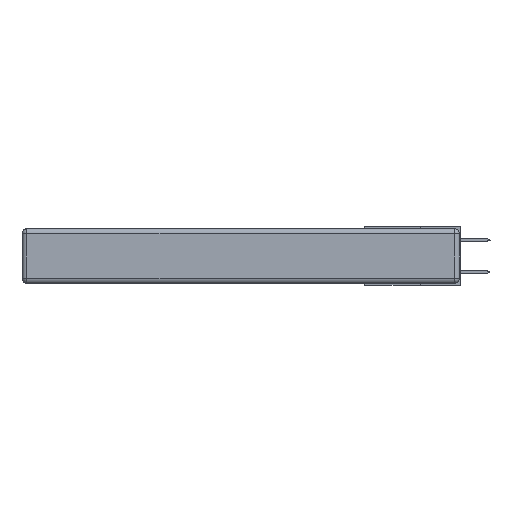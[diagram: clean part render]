
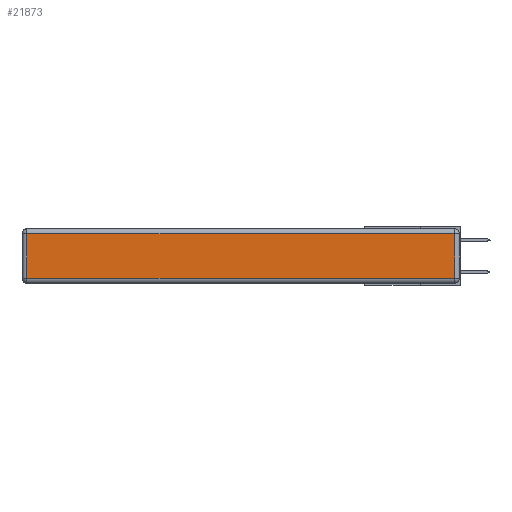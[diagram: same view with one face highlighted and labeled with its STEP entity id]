
A CAD part, left-side view. The second image highlights one B-rep face of the part: STEP entity #21873.
In plain terms, the highlighted planar face has unit normal (-1, 0, 0).
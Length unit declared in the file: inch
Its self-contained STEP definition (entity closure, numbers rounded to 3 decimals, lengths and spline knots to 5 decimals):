
#344 = DIRECTION ( 'NONE',  ( 0., -1., 0. ) ) ;
#1758 = CARTESIAN_POINT ( 'NONE',  ( 0., 2.72, -0.03 ) ) ;
#2579 = VECTOR ( 'NONE', #24734, 39.37008 ) ;
#2649 = CARTESIAN_POINT ( 'NONE',  ( 0., 2.75, -0.03 ) ) ;
#3263 = VECTOR ( 'NONE', #19631, 39.37008 ) ;
#4233 = VERTEX_POINT ( 'NONE', #17367 ) ;
#4449 = CARTESIAN_POINT ( 'NONE',  ( 0., 2.72, -0.313 ) ) ;
#5988 = ORIENTED_EDGE ( 'NONE', *, *, #15330, .T. ) ;
#6718 = DIRECTION ( 'NONE',  ( 0., 0., 1. ) ) ;
#6747 = DIRECTION ( 'NONE',  ( 0., 0., 1. ) ) ;
#8093 = AXIS2_PLACEMENT_3D ( 'NONE', #22631, #10865, #6718 ) ;
#8631 = EDGE_CURVE ( 'NONE', #15561, #10934, #18462, .T. ) ;
#10658 = ORIENTED_EDGE ( 'NONE', *, *, #12540, .T. ) ;
#10768 = LINE ( 'NONE', #16270, #16084 ) ;
#10865 = DIRECTION ( 'NONE',  ( -1., 0., 0. ) ) ;
#10934 = VERTEX_POINT ( 'NONE', #4449 ) ;
#12540 = EDGE_CURVE ( 'NONE', #10934, #23434, #10768, .T. ) ;
#13894 = LINE ( 'NONE', #24574, #16396 ) ;
#15330 = EDGE_CURVE ( 'NONE', #4233, #15561, #20598, .T. ) ;
#15541 = ORIENTED_EDGE ( 'NONE', *, *, #18241, .T. ) ;
#15561 = VERTEX_POINT ( 'NONE', #1758 ) ;
#15569 = CARTESIAN_POINT ( 'NONE',  ( 0., 2.72, -0.343 ) ) ;
#16084 = VECTOR ( 'NONE', #344, 39.37008 ) ;
#16270 = CARTESIAN_POINT ( 'NONE',  ( 0., 0., -0.313 ) ) ;
#16351 = EDGE_LOOP ( 'NONE', ( #10658, #15541, #5988, #24490 ) ) ;
#16396 = VECTOR ( 'NONE', #6747, 39.37008 ) ;
#16616 = CARTESIAN_POINT ( 'NONE',  ( 0., 0.03, -0.313 ) ) ;
#17212 = FACE_OUTER_BOUND ( 'NONE', #16351, .T. ) ;
#17367 = CARTESIAN_POINT ( 'NONE',  ( 0., 0.03, -0.03 ) ) ;
#18241 = EDGE_CURVE ( 'NONE', #23434, #4233, #13894, .T. ) ;
#18462 = LINE ( 'NONE', #15569, #3263 ) ;
#19631 = DIRECTION ( 'NONE',  ( 0., 0., -1. ) ) ;
#20598 = LINE ( 'NONE', #2649, #2579 ) ;
#21873 = ADVANCED_FACE ( 'NONE', ( #17212 ), #22803, .T. ) ;
#22631 = CARTESIAN_POINT ( 'NONE',  ( 0., 0., -0.343 ) ) ;
#22803 = PLANE ( 'NONE',  #8093 ) ;
#23434 = VERTEX_POINT ( 'NONE', #16616 ) ;
#24490 = ORIENTED_EDGE ( 'NONE', *, *, #8631, .T. ) ;
#24574 = CARTESIAN_POINT ( 'NONE',  ( 0., 0.03, -0.343 ) ) ;
#24734 = DIRECTION ( 'NONE',  ( 0., 1., 0. ) ) ;
